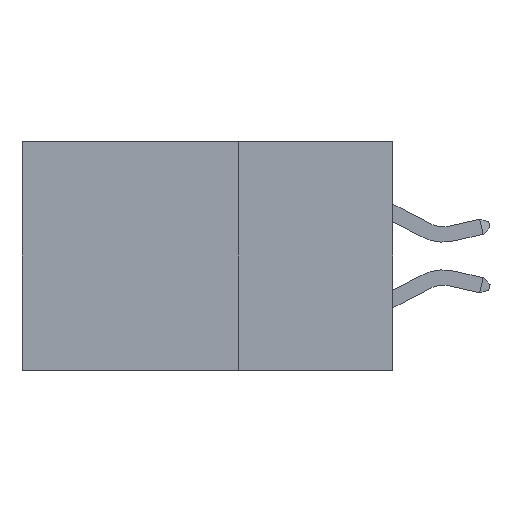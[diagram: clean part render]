
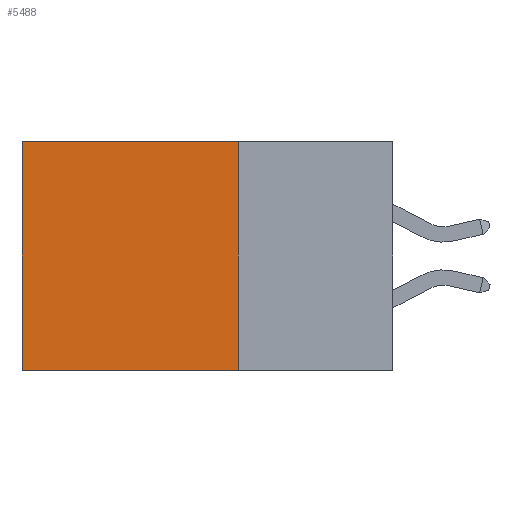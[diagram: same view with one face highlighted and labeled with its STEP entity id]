
A CAD part, left-side view. The second image highlights one B-rep face of the part: STEP entity #5488.
In plain terms, the highlighted planar face has unit normal (-1, 0, 0).
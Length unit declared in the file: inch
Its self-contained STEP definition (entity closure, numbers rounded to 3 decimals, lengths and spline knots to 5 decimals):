
#353 = VECTOR ( 'NONE', #9205, 39.37008 ) ;
#838 = LINE ( 'NONE', #5383, #9242 ) ;
#1104 = EDGE_LOOP ( 'NONE', ( #6494, #8516, #10685, #1538 ) ) ;
#1185 = FACE_OUTER_BOUND ( 'NONE', #1104, .T. ) ;
#1256 = EDGE_CURVE ( 'NONE', #2706, #4122, #7681, .T. ) ;
#1287 = VECTOR ( 'NONE', #7621, 39.37008 ) ;
#1538 = ORIENTED_EDGE ( 'NONE', *, *, #1591, .T. ) ;
#1591 = EDGE_CURVE ( 'NONE', #2706, #9541, #838, .T. ) ;
#2390 = CARTESIAN_POINT ( 'NONE',  ( 0.2875, 0.25, 0. ) ) ;
#2554 = CARTESIAN_POINT ( 'NONE',  ( 0.2875, 0.6, 0. ) ) ;
#2706 = VERTEX_POINT ( 'NONE', #11051 ) ;
#3306 = DIRECTION ( 'NONE',  ( 1., 0., 0. ) ) ;
#3434 = DIRECTION ( 'NONE',  ( 0., 0., -1. ) ) ;
#4122 = VERTEX_POINT ( 'NONE', #6247 ) ;
#4210 = AXIS2_PLACEMENT_3D ( 'NONE', #2390, #3306, #3434 ) ;
#4413 = EDGE_CURVE ( 'NONE', #9541, #12164, #10414, .T. ) ;
#4865 = DIRECTION ( 'NONE',  ( 0., 0., -1. ) ) ;
#5383 = CARTESIAN_POINT ( 'NONE',  ( 0.2875, 0.25, 0. ) ) ;
#5488 = ADVANCED_FACE ( 'NONE', ( #1185 ), #12328, .F. ) ;
#5683 = VECTOR ( 'NONE', #4865, 39.37008 ) ;
#6247 = CARTESIAN_POINT ( 'NONE',  ( 0.2875, 0.25, -0.37 ) ) ;
#6494 = ORIENTED_EDGE ( 'NONE', *, *, #4413, .T. ) ;
#7396 = DIRECTION ( 'NONE',  ( 0., 1., 0. ) ) ;
#7621 = DIRECTION ( 'NONE',  ( 0., 1., 0. ) ) ;
#7681 = LINE ( 'NONE', #8030, #353 ) ;
#7821 = EDGE_CURVE ( 'NONE', #4122, #12164, #12521, .T. ) ;
#8030 = CARTESIAN_POINT ( 'NONE',  ( 0.2875, 0.25, 0. ) ) ;
#8516 = ORIENTED_EDGE ( 'NONE', *, *, #7821, .F. ) ;
#9205 = DIRECTION ( 'NONE',  ( 0., 0., -1. ) ) ;
#9242 = VECTOR ( 'NONE', #7396, 39.37008 ) ;
#9483 = CARTESIAN_POINT ( 'NONE',  ( 0.2875, 0.6, -0.37 ) ) ;
#9541 = VERTEX_POINT ( 'NONE', #2554 ) ;
#9955 = CARTESIAN_POINT ( 'NONE',  ( 0.2875, 0.6, 0. ) ) ;
#10414 = LINE ( 'NONE', #9955, #5683 ) ;
#10685 = ORIENTED_EDGE ( 'NONE', *, *, #1256, .F. ) ;
#11051 = CARTESIAN_POINT ( 'NONE',  ( 0.2875, 0.25, 0. ) ) ;
#11634 = CARTESIAN_POINT ( 'NONE',  ( 0.2875, 0.25, -0.37 ) ) ;
#12164 = VERTEX_POINT ( 'NONE', #9483 ) ;
#12328 = PLANE ( 'NONE',  #4210 ) ;
#12521 = LINE ( 'NONE', #11634, #1287 ) ;
